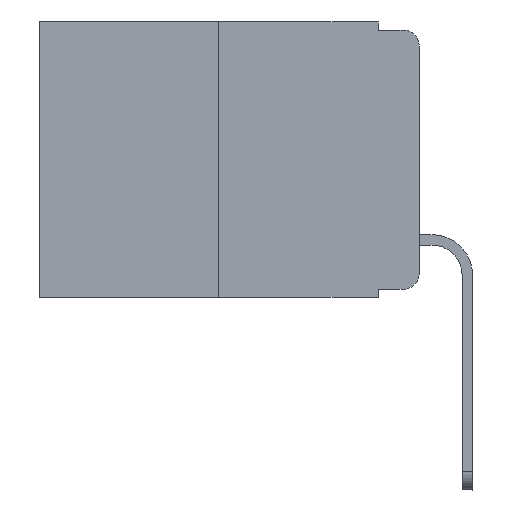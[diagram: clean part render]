
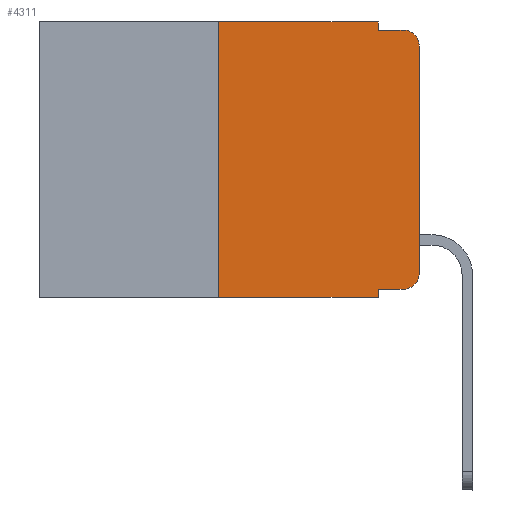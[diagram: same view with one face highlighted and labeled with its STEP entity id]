
A CAD part, left-side view. The second image highlights one B-rep face of the part: STEP entity #4311.
In plain terms, the highlighted planar face has unit normal (-1, 0, 0).
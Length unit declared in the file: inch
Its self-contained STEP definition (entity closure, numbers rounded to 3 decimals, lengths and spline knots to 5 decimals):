
#458 = VERTEX_POINT ( 'NONE', #2979 ) ;
#869 = VECTOR ( 'NONE', #15461, 39.37008 ) ;
#1110 = LINE ( 'NONE', #13897, #9728 ) ;
#1181 = CARTESIAN_POINT ( 'NONE',  ( 0., 0.02, -0.333 ) ) ;
#1208 = DIRECTION ( 'NONE',  ( 0., 0., -1. ) ) ;
#1830 = CARTESIAN_POINT ( 'NONE',  ( 0., 0.051, -0.343 ) ) ;
#1908 = DIRECTION ( 'NONE',  ( 0., -1., 0. ) ) ;
#2137 = DIRECTION ( 'NONE',  ( 0., 0., 1. ) ) ;
#2878 = LINE ( 'NONE', #20121, #869 ) ;
#2979 = CARTESIAN_POINT ( 'NONE',  ( 0., 0.25, 0. ) ) ;
#3108 = DIRECTION ( 'NONE',  ( 0., 0., -1. ) ) ;
#3457 = LINE ( 'NONE', #14600, #4412 ) ;
#3636 = VERTEX_POINT ( 'NONE', #1830 ) ;
#3677 = CARTESIAN_POINT ( 'NONE',  ( 0., 0., -0.313 ) ) ;
#4156 = DIRECTION ( 'NONE',  ( 0., 0., -1. ) ) ;
#4292 = DIRECTION ( 'NONE',  ( 0., -1., 0. ) ) ;
#4311 = ADVANCED_FACE ( 'NONE', ( #12122 ), #5705, .F. ) ;
#4334 = CARTESIAN_POINT ( 'NONE',  ( 0., 0.051, 0. ) ) ;
#4372 = EDGE_CURVE ( 'NONE', #10267, #13338, #5692, .T. ) ;
#4412 = VECTOR ( 'NONE', #1908, 39.37008 ) ;
#5120 = ORIENTED_EDGE ( 'NONE', *, *, #20394, .F. ) ;
#5123 = ORIENTED_EDGE ( 'NONE', *, *, #14834, .F. ) ;
#5603 = CARTESIAN_POINT ( 'NONE',  ( 0., 0.473, 0. ) ) ;
#5692 = CIRCLE ( 'NONE', #17243, 0.02 ) ;
#5705 = PLANE ( 'NONE',  #13920 ) ;
#5777 = CIRCLE ( 'NONE', #7412, 0.02 ) ;
#6201 = DIRECTION ( 'NONE',  ( -1., 0., 0. ) ) ;
#6618 = EDGE_CURVE ( 'NONE', #6899, #3636, #7430, .T. ) ;
#6856 = CARTESIAN_POINT ( 'NONE',  ( 0., 0., -0.03 ) ) ;
#6899 = VERTEX_POINT ( 'NONE', #14758 ) ;
#7140 = EDGE_CURVE ( 'NONE', #6899, #13407, #3457, .T. ) ;
#7180 = DIRECTION ( 'NONE',  ( -1., 0., 0. ) ) ;
#7293 = VECTOR ( 'NONE', #8994, 39.37008 ) ;
#7342 = ORIENTED_EDGE ( 'NONE', *, *, #6618, .F. ) ;
#7412 = AXIS2_PLACEMENT_3D ( 'NONE', #15334, #7180, #1208 ) ;
#7430 = LINE ( 'NONE', #13754, #15183 ) ;
#8375 = CARTESIAN_POINT ( 'NONE',  ( 0., 0.25, -0.343 ) ) ;
#8575 = ORIENTED_EDGE ( 'NONE', *, *, #13037, .T. ) ;
#8994 = DIRECTION ( 'NONE',  ( 0., -1., 0. ) ) ;
#9021 = EDGE_CURVE ( 'NONE', #458, #10831, #10469, .T. ) ;
#9509 = CARTESIAN_POINT ( 'NONE',  ( 0., 0.02, -0.03 ) ) ;
#9728 = VECTOR ( 'NONE', #4292, 39.37008 ) ;
#10267 = VERTEX_POINT ( 'NONE', #6856 ) ;
#10469 = LINE ( 'NONE', #12010, #7293 ) ;
#10485 = CARTESIAN_POINT ( 'NONE',  ( 0., 0.02, -0.01 ) ) ;
#10514 = EDGE_LOOP ( 'NONE', ( #15622, #13960, #11793, #5120, #14935, #5123, #10817, #7342, #17685, #8575 ) ) ;
#10796 = LINE ( 'NONE', #12337, #16740 ) ;
#10817 = ORIENTED_EDGE ( 'NONE', *, *, #16661, .T. ) ;
#10831 = VERTEX_POINT ( 'NONE', #4334 ) ;
#11213 = EDGE_CURVE ( 'NONE', #11592, #10267, #2878, .T. ) ;
#11500 = VECTOR ( 'NONE', #19967, 39.37008 ) ;
#11592 = VERTEX_POINT ( 'NONE', #3677 ) ;
#11793 = ORIENTED_EDGE ( 'NONE', *, *, #13021, .F. ) ;
#12010 = CARTESIAN_POINT ( 'NONE',  ( 0., 0.473, 0. ) ) ;
#12014 = DIRECTION ( 'NONE',  ( 1., 0., 0. ) ) ;
#12122 = FACE_OUTER_BOUND ( 'NONE', #10514, .T. ) ;
#12302 = DIRECTION ( 'NONE',  ( 0., 0., -1. ) ) ;
#12337 = CARTESIAN_POINT ( 'NONE',  ( 0., 0.051, 0. ) ) ;
#12511 = VERTEX_POINT ( 'NONE', #15465 ) ;
#13021 = EDGE_CURVE ( 'NONE', #12511, #13338, #1110, .T. ) ;
#13037 = EDGE_CURVE ( 'NONE', #13407, #11592, #5777, .T. ) ;
#13338 = VERTEX_POINT ( 'NONE', #10485 ) ;
#13407 = VERTEX_POINT ( 'NONE', #1181 ) ;
#13679 = CARTESIAN_POINT ( 'NONE',  ( 0., 0.473, -0.343 ) ) ;
#13754 = CARTESIAN_POINT ( 'NONE',  ( 0., 0.051, 0. ) ) ;
#13891 = DIRECTION ( 'NONE',  ( 0., 0., -1. ) ) ;
#13897 = CARTESIAN_POINT ( 'NONE',  ( 0., 0.051, -0.01 ) ) ;
#13920 = AXIS2_PLACEMENT_3D ( 'NONE', #5603, #12014, #4156 ) ;
#13960 = ORIENTED_EDGE ( 'NONE', *, *, #4372, .T. ) ;
#14600 = CARTESIAN_POINT ( 'NONE',  ( 0., 0.051, -0.333 ) ) ;
#14758 = CARTESIAN_POINT ( 'NONE',  ( 0., 0.051, -0.333 ) ) ;
#14834 = EDGE_CURVE ( 'NONE', #18225, #458, #19484, .T. ) ;
#14935 = ORIENTED_EDGE ( 'NONE', *, *, #9021, .F. ) ;
#15183 = VECTOR ( 'NONE', #12302, 39.37008 ) ;
#15334 = CARTESIAN_POINT ( 'NONE',  ( 0., 0.02, -0.313 ) ) ;
#15397 = VECTOR ( 'NONE', #2137, 39.37008 ) ;
#15424 = LINE ( 'NONE', #13679, #11500 ) ;
#15461 = DIRECTION ( 'NONE',  ( 0., 0., 1. ) ) ;
#15465 = CARTESIAN_POINT ( 'NONE',  ( 0., 0.051, -0.01 ) ) ;
#15622 = ORIENTED_EDGE ( 'NONE', *, *, #11213, .T. ) ;
#16282 = CARTESIAN_POINT ( 'NONE',  ( 0., 0.25, 0. ) ) ;
#16661 = EDGE_CURVE ( 'NONE', #18225, #3636, #15424, .T. ) ;
#16740 = VECTOR ( 'NONE', #13891, 39.37008 ) ;
#17243 = AXIS2_PLACEMENT_3D ( 'NONE', #9509, #6201, #3108 ) ;
#17685 = ORIENTED_EDGE ( 'NONE', *, *, #7140, .T. ) ;
#18225 = VERTEX_POINT ( 'NONE', #8375 ) ;
#19484 = LINE ( 'NONE', #16282, #15397 ) ;
#19967 = DIRECTION ( 'NONE',  ( 0., -1., 0. ) ) ;
#20121 = CARTESIAN_POINT ( 'NONE',  ( 0., 0., 0. ) ) ;
#20394 = EDGE_CURVE ( 'NONE', #10831, #12511, #10796, .T. ) ;
